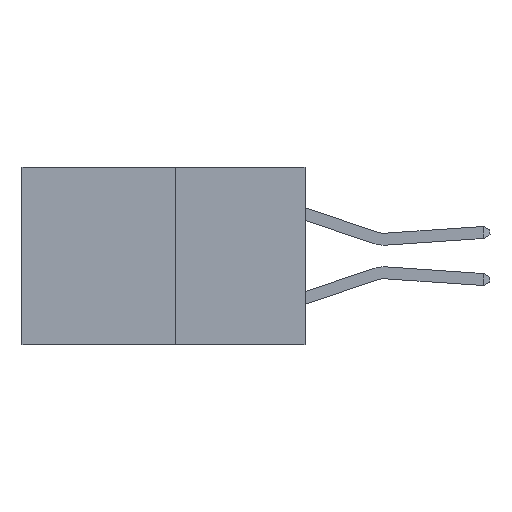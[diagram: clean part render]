
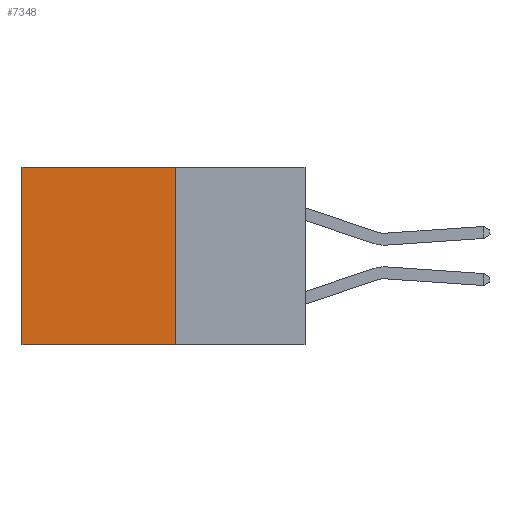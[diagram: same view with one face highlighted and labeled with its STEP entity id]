
A CAD part, left-side view. The second image highlights one B-rep face of the part: STEP entity #7348.
In plain terms, the highlighted planar face has unit normal (-1, 0, 0).
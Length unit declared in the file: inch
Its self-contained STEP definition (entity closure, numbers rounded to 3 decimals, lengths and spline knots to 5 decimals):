
#90 = VERTEX_POINT ( 'NONE', #5249 ) ;
#965 = EDGE_CURVE ( 'NONE', #90, #3561, #5262, .T. ) ;
#1102 = ORIENTED_EDGE ( 'NONE', *, *, #965, .T. ) ;
#1523 = FACE_OUTER_BOUND ( 'NONE', #11072, .T. ) ;
#1608 = ORIENTED_EDGE ( 'NONE', *, *, #1688, .T. ) ;
#1647 = EDGE_CURVE ( 'NONE', #4500, #3561, #10759, .T. ) ;
#1688 = EDGE_CURVE ( 'NONE', #8388, #90, #3341, .T. ) ;
#1869 = DIRECTION ( 'NONE',  ( 0., 0., -1. ) ) ;
#1970 = CARTESIAN_POINT ( 'NONE',  ( 0.277, 0.27, 0. ) ) ;
#2309 = CARTESIAN_POINT ( 'NONE',  ( 0.277, 0.59, -0.37 ) ) ;
#2845 = DIRECTION ( 'NONE',  ( 1., 0., 0. ) ) ;
#3109 = EDGE_CURVE ( 'NONE', #8388, #4500, #9854, .T. ) ;
#3341 = LINE ( 'NONE', #4262, #5726 ) ;
#3561 = VERTEX_POINT ( 'NONE', #5882 ) ;
#3960 = VECTOR ( 'NONE', #4565, 39.37008 ) ;
#4227 = DIRECTION ( 'NONE',  ( 0., 1., 0. ) ) ;
#4262 = CARTESIAN_POINT ( 'NONE',  ( 0.277, 0.27, 0. ) ) ;
#4500 = VERTEX_POINT ( 'NONE', #7352 ) ;
#4565 = DIRECTION ( 'NONE',  ( 0., 1., 0. ) ) ;
#4583 = CARTESIAN_POINT ( 'NONE',  ( 0.277, 0.27, -0.37 ) ) ;
#5249 = CARTESIAN_POINT ( 'NONE',  ( 0.277, 0.59, 0. ) ) ;
#5262 = LINE ( 'NONE', #2309, #9725 ) ;
#5279 = VECTOR ( 'NONE', #8661, 39.37008 ) ;
#5726 = VECTOR ( 'NONE', #4227, 39.37008 ) ;
#5882 = CARTESIAN_POINT ( 'NONE',  ( 0.277, 0.59, -0.37 ) ) ;
#7313 = PLANE ( 'NONE',  #8230 ) ;
#7348 = ADVANCED_FACE ( 'NONE', ( #1523 ), #7313, .F. ) ;
#7352 = CARTESIAN_POINT ( 'NONE',  ( 0.277, 0.27, -0.37 ) ) ;
#8199 = CARTESIAN_POINT ( 'NONE',  ( 0.277, 0.27, -0.37 ) ) ;
#8230 = AXIS2_PLACEMENT_3D ( 'NONE', #8199, #2845, #9048 ) ;
#8388 = VERTEX_POINT ( 'NONE', #1970 ) ;
#8661 = DIRECTION ( 'NONE',  ( 0., 0., -1. ) ) ;
#9048 = DIRECTION ( 'NONE',  ( 0., 0., -1. ) ) ;
#9490 = CARTESIAN_POINT ( 'NONE',  ( 0.277, 0.27, -0.37 ) ) ;
#9721 = ORIENTED_EDGE ( 'NONE', *, *, #3109, .F. ) ;
#9725 = VECTOR ( 'NONE', #1869, 39.37008 ) ;
#9854 = LINE ( 'NONE', #9490, #5279 ) ;
#10602 = ORIENTED_EDGE ( 'NONE', *, *, #1647, .F. ) ;
#10759 = LINE ( 'NONE', #4583, #3960 ) ;
#11072 = EDGE_LOOP ( 'NONE', ( #1102, #10602, #9721, #1608 ) ) ;
